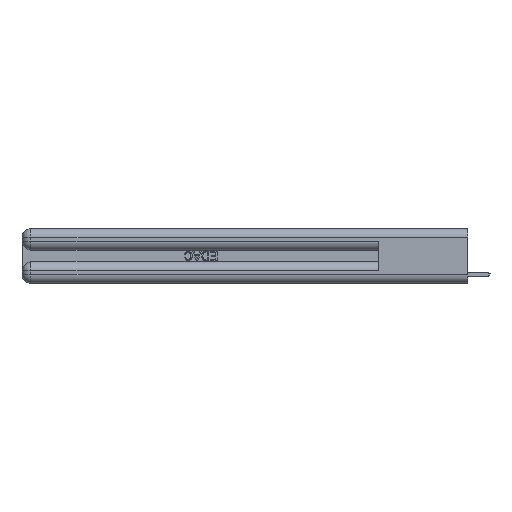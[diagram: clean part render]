
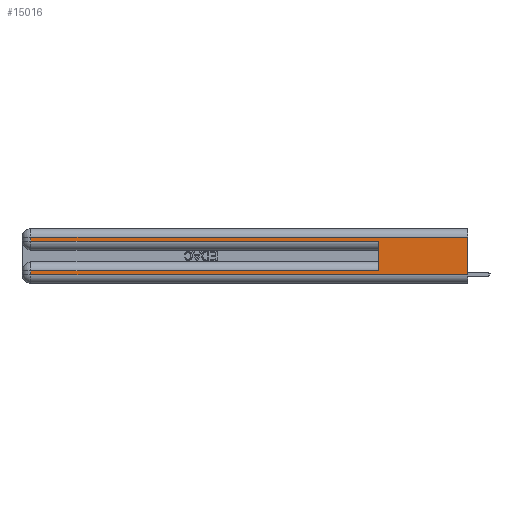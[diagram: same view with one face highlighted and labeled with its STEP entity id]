
A CAD part, left-side view. The second image highlights one B-rep face of the part: STEP entity #15016.
In plain terms, the highlighted planar face has unit normal (-1, 0, 0).
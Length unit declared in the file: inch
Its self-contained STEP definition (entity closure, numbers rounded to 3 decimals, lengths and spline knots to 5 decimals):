
#1672 = ORIENTED_EDGE ( 'NONE', *, *, #11175, .T. ) ;
#2576 = VECTOR ( 'NONE', #22553, 39.37008 ) ;
#2606 = LINE ( 'NONE', #8468, #8073 ) ;
#3774 = VERTEX_POINT ( 'NONE', #5624 ) ;
#3876 = DIRECTION ( 'NONE',  ( 0., 0., -1. ) ) ;
#4462 = VECTOR ( 'NONE', #20633, 39.37008 ) ;
#5624 = CARTESIAN_POINT ( 'NONE',  ( 0., 2.94, 0.085 ) ) ;
#5970 = EDGE_CURVE ( 'NONE', #33294, #15103, #21647, .T. ) ;
#6039 = DIRECTION ( 'NONE',  ( 1., 0., 0. ) ) ;
#6441 = CARTESIAN_POINT ( 'NONE',  ( 0., 0.6, 0.085 ) ) ;
#6800 = VERTEX_POINT ( 'NONE', #24526 ) ;
#7438 = CARTESIAN_POINT ( 'NONE',  ( 0., 0.6, 0.145 ) ) ;
#8073 = VECTOR ( 'NONE', #29954, 39.37008 ) ;
#8335 = CARTESIAN_POINT ( 'NONE',  ( 0., 0., 0.37 ) ) ;
#8347 = CARTESIAN_POINT ( 'NONE',  ( 0., 2.94, 0.31 ) ) ;
#8468 = CARTESIAN_POINT ( 'NONE',  ( 0., 0., 0.31 ) ) ;
#8513 = DIRECTION ( 'NONE',  ( 0., 0., -1. ) ) ;
#9042 = FACE_OUTER_BOUND ( 'NONE', #22364, .T. ) ;
#9149 = LINE ( 'NONE', #20342, #20498 ) ;
#9675 = ORIENTED_EDGE ( 'NONE', *, *, #5970, .F. ) ;
#9939 = VECTOR ( 'NONE', #3876, 39.37008 ) ;
#10374 = EDGE_CURVE ( 'NONE', #15072, #6800, #34299, .T. ) ;
#10448 = VECTOR ( 'NONE', #26341, 39.37008 ) ;
#11175 = EDGE_CURVE ( 'NONE', #33294, #3774, #22701, .T. ) ;
#12046 = LINE ( 'NONE', #22892, #2576 ) ;
#12774 = EDGE_CURVE ( 'NONE', #15044, #15103, #9149, .T. ) ;
#13359 = ORIENTED_EDGE ( 'NONE', *, *, #34633, .F. ) ;
#13633 = EDGE_CURVE ( 'NONE', #17157, #21239, #2606, .T. ) ;
#13877 = ORIENTED_EDGE ( 'NONE', *, *, #10374, .T. ) ;
#14020 = CARTESIAN_POINT ( 'NONE',  ( 0., 2.94, 0.06 ) ) ;
#15016 = ADVANCED_FACE ( 'NONE', ( #9042 ), #20536, .F. ) ;
#15044 = VERTEX_POINT ( 'NONE', #19349 ) ;
#15072 = VERTEX_POINT ( 'NONE', #14020 ) ;
#15103 = VERTEX_POINT ( 'NONE', #30346 ) ;
#15503 = CARTESIAN_POINT ( 'NONE',  ( 0., 2.94, 0.37 ) ) ;
#17157 = VERTEX_POINT ( 'NONE', #25088 ) ;
#18893 = AXIS2_PLACEMENT_3D ( 'NONE', #31356, #6039, #8513 ) ;
#19349 = CARTESIAN_POINT ( 'NONE',  ( 0., 2.94, 0.285 ) ) ;
#19448 = ORIENTED_EDGE ( 'NONE', *, *, #20685, .T. ) ;
#20197 = EDGE_CURVE ( 'NONE', #21239, #15044, #12046, .T. ) ;
#20342 = CARTESIAN_POINT ( 'NONE',  ( 0., 0., 0.285 ) ) ;
#20498 = VECTOR ( 'NONE', #26011, 39.37008 ) ;
#20536 = PLANE ( 'NONE',  #18893 ) ;
#20633 = DIRECTION ( 'NONE',  ( 0., -1., 0. ) ) ;
#20685 = EDGE_CURVE ( 'NONE', #3774, #15072, #21033, .T. ) ;
#20815 = ORIENTED_EDGE ( 'NONE', *, *, #20197, .T. ) ;
#21033 = LINE ( 'NONE', #15503, #10448 ) ;
#21239 = VERTEX_POINT ( 'NONE', #8347 ) ;
#21647 = LINE ( 'NONE', #7438, #29878 ) ;
#22364 = EDGE_LOOP ( 'NONE', ( #13359, #24848, #20815, #34147, #9675, #1672, #19448, #13877 ) ) ;
#22553 = DIRECTION ( 'NONE',  ( 0., 0., -1. ) ) ;
#22701 = LINE ( 'NONE', #28539, #33467 ) ;
#22892 = CARTESIAN_POINT ( 'NONE',  ( 0., 2.94, 0.37 ) ) ;
#23031 = DIRECTION ( 'NONE',  ( 0., 1., 0. ) ) ;
#23463 = CARTESIAN_POINT ( 'NONE',  ( 0., 0., 0.06 ) ) ;
#24526 = CARTESIAN_POINT ( 'NONE',  ( 0., 0., 0.06 ) ) ;
#24848 = ORIENTED_EDGE ( 'NONE', *, *, #13633, .T. ) ;
#25088 = CARTESIAN_POINT ( 'NONE',  ( 0., 0., 0.31 ) ) ;
#26011 = DIRECTION ( 'NONE',  ( 0., -1., 0. ) ) ;
#26341 = DIRECTION ( 'NONE',  ( 0., 0., -1. ) ) ;
#28539 = CARTESIAN_POINT ( 'NONE',  ( 0., 0., 0.085 ) ) ;
#29878 = VECTOR ( 'NONE', #34787, 39.37008 ) ;
#29954 = DIRECTION ( 'NONE',  ( 0., 1., 0. ) ) ;
#30346 = CARTESIAN_POINT ( 'NONE',  ( 0., 0.6, 0.285 ) ) ;
#31356 = CARTESIAN_POINT ( 'NONE',  ( 0., 0., 0.37 ) ) ;
#32668 = LINE ( 'NONE', #8335, #9939 ) ;
#33294 = VERTEX_POINT ( 'NONE', #6441 ) ;
#33467 = VECTOR ( 'NONE', #23031, 39.37008 ) ;
#34147 = ORIENTED_EDGE ( 'NONE', *, *, #12774, .T. ) ;
#34299 = LINE ( 'NONE', #23463, #4462 ) ;
#34633 = EDGE_CURVE ( 'NONE', #17157, #6800, #32668, .T. ) ;
#34787 = DIRECTION ( 'NONE',  ( 0., 0., 1. ) ) ;
